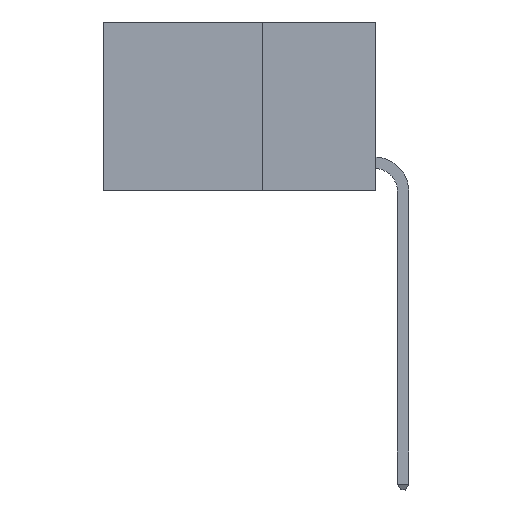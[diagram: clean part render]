
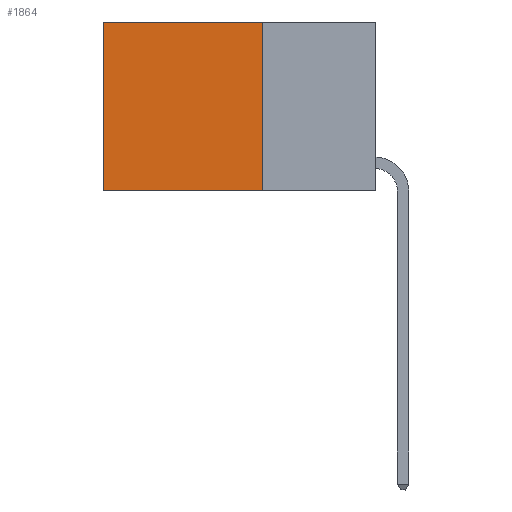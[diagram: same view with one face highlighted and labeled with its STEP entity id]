
A CAD part, left-side view. The second image highlights one B-rep face of the part: STEP entity #1864.
In plain terms, the highlighted planar face has unit normal (-1, 0, 0).
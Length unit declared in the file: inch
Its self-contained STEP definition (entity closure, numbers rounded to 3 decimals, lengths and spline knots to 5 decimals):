
#109 = VERTEX_POINT ( 'NONE', #2927 ) ;
#522 = CARTESIAN_POINT ( 'NONE',  ( 0.2625, 0.25, 0. ) ) ;
#1169 = EDGE_CURVE ( 'NONE', #6316, #7726, #5352, .T. ) ;
#1303 = VECTOR ( 'NONE', #3368, 39.37008 ) ;
#1510 = AXIS2_PLACEMENT_3D ( 'NONE', #4437, #11609, #8461 ) ;
#1676 = LINE ( 'NONE', #7865, #1303 ) ;
#1813 = ORIENTED_EDGE ( 'NONE', *, *, #12340, .T. ) ;
#1864 = ADVANCED_FACE ( 'NONE', ( #14199 ), #12818, .F. ) ;
#2128 = LINE ( 'NONE', #11367, #10669 ) ;
#2927 = CARTESIAN_POINT ( 'NONE',  ( 0.2625, 0.6, -0.37 ) ) ;
#3368 = DIRECTION ( 'NONE',  ( 0., 1., 0. ) ) ;
#4343 = LINE ( 'NONE', #6157, #9919 ) ;
#4437 = CARTESIAN_POINT ( 'NONE',  ( 0.2625, 0.25, 0. ) ) ;
#5219 = ORIENTED_EDGE ( 'NONE', *, *, #13768, .T. ) ;
#5249 = CARTESIAN_POINT ( 'NONE',  ( 0.2625, 0.25, -0.37 ) ) ;
#5352 = LINE ( 'NONE', #9646, #13935 ) ;
#6157 = CARTESIAN_POINT ( 'NONE',  ( 0.2625, 0.25, 0. ) ) ;
#6316 = VERTEX_POINT ( 'NONE', #522 ) ;
#7328 = DIRECTION ( 'NONE',  ( 0., 1., 0. ) ) ;
#7687 = VERTEX_POINT ( 'NONE', #11421 ) ;
#7726 = VERTEX_POINT ( 'NONE', #5249 ) ;
#7865 = CARTESIAN_POINT ( 'NONE',  ( 0.2625, 0.25, -0.37 ) ) ;
#8461 = DIRECTION ( 'NONE',  ( 0., 0., -1. ) ) ;
#8864 = DIRECTION ( 'NONE',  ( 0., 0., -1. ) ) ;
#9052 = ORIENTED_EDGE ( 'NONE', *, *, #1169, .F. ) ;
#9520 = EDGE_CURVE ( 'NONE', #7726, #109, #1676, .T. ) ;
#9646 = CARTESIAN_POINT ( 'NONE',  ( 0.2625, 0.25, 0. ) ) ;
#9919 = VECTOR ( 'NONE', #7328, 39.37008 ) ;
#10329 = EDGE_LOOP ( 'NONE', ( #1813, #12869, #9052, #5219 ) ) ;
#10669 = VECTOR ( 'NONE', #13642, 39.37008 ) ;
#11367 = CARTESIAN_POINT ( 'NONE',  ( 0.2625, 0.6, 0. ) ) ;
#11421 = CARTESIAN_POINT ( 'NONE',  ( 0.2625, 0.6, 0. ) ) ;
#11609 = DIRECTION ( 'NONE',  ( 1., 0., 0. ) ) ;
#12340 = EDGE_CURVE ( 'NONE', #7687, #109, #2128, .T. ) ;
#12818 = PLANE ( 'NONE',  #1510 ) ;
#12869 = ORIENTED_EDGE ( 'NONE', *, *, #9520, .F. ) ;
#13642 = DIRECTION ( 'NONE',  ( 0., 0., -1. ) ) ;
#13768 = EDGE_CURVE ( 'NONE', #6316, #7687, #4343, .T. ) ;
#13935 = VECTOR ( 'NONE', #8864, 39.37008 ) ;
#14199 = FACE_OUTER_BOUND ( 'NONE', #10329, .T. ) ;
